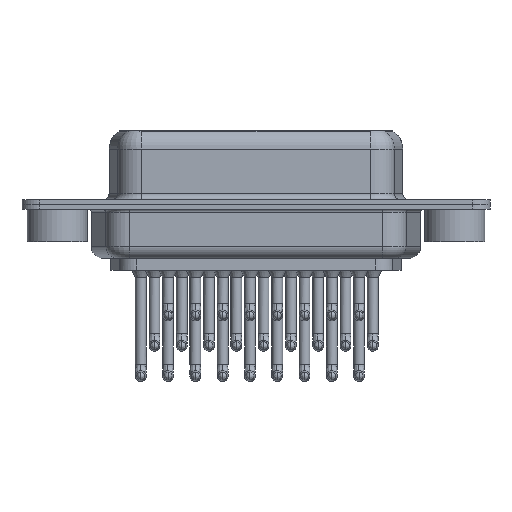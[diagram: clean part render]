
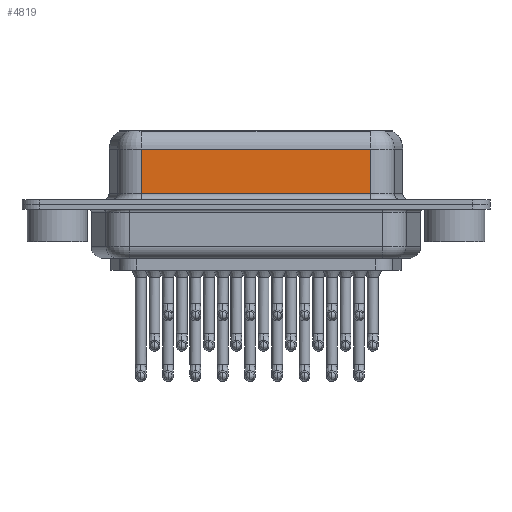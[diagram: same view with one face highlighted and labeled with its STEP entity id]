
A CAD part, front view. The second image highlights one B-rep face of the part: STEP entity #4819.
In plain terms, the highlighted planar face has unit normal (0, -1, 0).
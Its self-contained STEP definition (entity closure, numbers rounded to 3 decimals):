
#450 = VECTOR ( 'NONE', #18625, 1000. ) ;
#692 = VERTEX_POINT ( 'NONE', #11705 ) ;
#1657 = LINE ( 'NONE', #15929, #20650 ) ;
#2707 = EDGE_CURVE ( 'NONE', #10361, #692, #23716, .T. ) ;
#2909 = DIRECTION ( 'NONE',  ( 1., 0., 0. ) ) ;
#3550 = CARTESIAN_POINT ( 'NONE',  ( 7.038, -3.95, 4.65 ) ) ;
#3637 = CARTESIAN_POINT ( 'NONE',  ( 26.262, -3.95, 0.9 ) ) ;
#4117 = VERTEX_POINT ( 'NONE', #3637 ) ;
#4819 = ADVANCED_FACE ( 'NONE', ( #13532 ), #19950, .F. ) ;
#5758 = ORIENTED_EDGE ( 'NONE', *, *, #2707, .T. ) ;
#7579 = EDGE_CURVE ( 'NONE', #19359, #10361, #1657, .T. ) ;
#7725 = ORIENTED_EDGE ( 'NONE', *, *, #7579, .T. ) ;
#8208 = DIRECTION ( 'NONE',  ( 0., 0., -1. ) ) ;
#8386 = EDGE_LOOP ( 'NONE', ( #19947, #7725, #5758, #15695 ) ) ;
#8445 = CARTESIAN_POINT ( 'NONE',  ( 26.262, -3.95, 4.65 ) ) ;
#8624 = DIRECTION ( 'NONE',  ( -1., 0., 0. ) ) ;
#8957 = VECTOR ( 'NONE', #8208, 1000. ) ;
#9074 = DIRECTION ( 'NONE',  ( -1., 0., 0. ) ) ;
#10124 = EDGE_CURVE ( 'NONE', #692, #4117, #19989, .T. ) ;
#10196 = VECTOR ( 'NONE', #2909, 1000. ) ;
#10272 = DIRECTION ( 'NONE',  ( 0., 1., 0. ) ) ;
#10361 = VERTEX_POINT ( 'NONE', #3550 ) ;
#11705 = CARTESIAN_POINT ( 'NONE',  ( 7.038, -3.95, 0.9 ) ) ;
#11748 = EDGE_CURVE ( 'NONE', #19359, #4117, #22533, .T. ) ;
#13532 = FACE_OUTER_BOUND ( 'NONE', #8386, .T. ) ;
#13935 = CARTESIAN_POINT ( 'NONE',  ( 26.262, -3.95, 0.9 ) ) ;
#14332 = AXIS2_PLACEMENT_3D ( 'NONE', #20122, #10272, #9074 ) ;
#15695 = ORIENTED_EDGE ( 'NONE', *, *, #10124, .T. ) ;
#15929 = CARTESIAN_POINT ( 'NONE',  ( 26.262, -3.95, 4.65 ) ) ;
#18625 = DIRECTION ( 'NONE',  ( 0., 0., -1. ) ) ;
#19230 = CARTESIAN_POINT ( 'NONE',  ( 26.262, -3.95, 6.4 ) ) ;
#19359 = VERTEX_POINT ( 'NONE', #8445 ) ;
#19694 = CARTESIAN_POINT ( 'NONE',  ( 7.038, -3.95, 6.4 ) ) ;
#19947 = ORIENTED_EDGE ( 'NONE', *, *, #11748, .F. ) ;
#19950 = PLANE ( 'NONE',  #14332 ) ;
#19989 = LINE ( 'NONE', #13935, #10196 ) ;
#20122 = CARTESIAN_POINT ( 'NONE',  ( 26.262, -3.95, 6.4 ) ) ;
#20650 = VECTOR ( 'NONE', #8624, 1000. ) ;
#22533 = LINE ( 'NONE', #19230, #8957 ) ;
#23716 = LINE ( 'NONE', #19694, #450 ) ;
